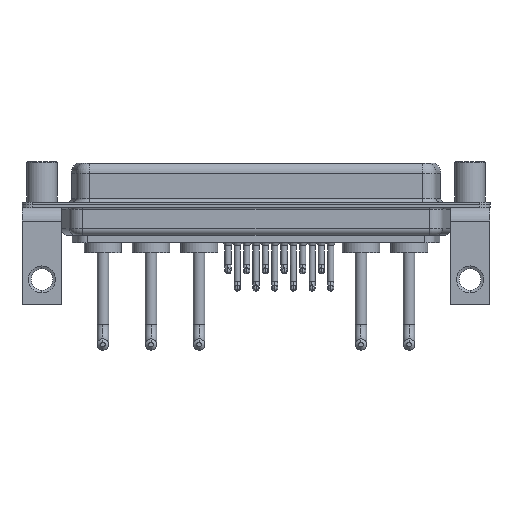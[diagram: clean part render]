
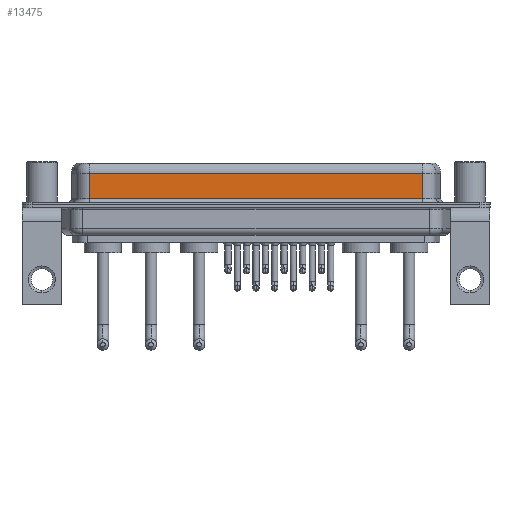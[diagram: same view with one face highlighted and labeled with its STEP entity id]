
A CAD part, front view. The second image highlights one B-rep face of the part: STEP entity #13475.
In plain terms, the highlighted planar face has unit normal (0, -1, 0).
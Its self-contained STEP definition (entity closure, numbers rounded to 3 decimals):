
#339 = VERTEX_POINT ( 'NONE', #3118 ) ;
#616 = DIRECTION ( 'NONE',  ( -1., 0., 0. ) ) ;
#667 = ORIENTED_EDGE ( 'NONE', *, *, #9464, .T. ) ;
#1464 = VECTOR ( 'NONE', #3838, 1000. ) ;
#2189 = LINE ( 'NONE', #9022, #3500 ) ;
#2222 = EDGE_CURVE ( 'NONE', #6596, #19165, #9717, .T. ) ;
#2508 = AXIS2_PLACEMENT_3D ( 'NONE', #5162, #19135, #3437 ) ;
#3118 = CARTESIAN_POINT ( 'NONE',  ( 7.038, -3.95, 4.65 ) ) ;
#3431 = EDGE_CURVE ( 'NONE', #14844, #19165, #19658, .T. ) ;
#3437 = DIRECTION ( 'NONE',  ( 0., 0., 1. ) ) ;
#3500 = VECTOR ( 'NONE', #616, 1000. ) ;
#3838 = DIRECTION ( 'NONE',  ( 1., 0., 0. ) ) ;
#5162 = CARTESIAN_POINT ( 'NONE',  ( 56.462, -3.95, 6.4 ) ) ;
#6596 = VERTEX_POINT ( 'NONE', #10594 ) ;
#6898 = CARTESIAN_POINT ( 'NONE',  ( 7.038, -3.95, 0.9 ) ) ;
#7156 = EDGE_LOOP ( 'NONE', ( #17201, #18753, #667, #19845 ) ) ;
#8074 = EDGE_CURVE ( 'NONE', #6596, #339, #2189, .T. ) ;
#9022 = CARTESIAN_POINT ( 'NONE',  ( 56.462, -3.95, 4.65 ) ) ;
#9261 = LINE ( 'NONE', #10861, #20850 ) ;
#9464 = EDGE_CURVE ( 'NONE', #339, #14844, #9261, .T. ) ;
#9717 = LINE ( 'NONE', #16739, #19604 ) ;
#10594 = CARTESIAN_POINT ( 'NONE',  ( 56.462, -3.95, 4.65 ) ) ;
#10861 = CARTESIAN_POINT ( 'NONE',  ( 7.038, -3.95, 6.4 ) ) ;
#12096 = PLANE ( 'NONE',  #2508 ) ;
#12380 = CARTESIAN_POINT ( 'NONE',  ( 56.462, -3.95, 0.9 ) ) ;
#13072 = DIRECTION ( 'NONE',  ( 0., 0., -1. ) ) ;
#13475 = ADVANCED_FACE ( 'NONE', ( #21288 ), #12096, .F. ) ;
#14844 = VERTEX_POINT ( 'NONE', #6898 ) ;
#16739 = CARTESIAN_POINT ( 'NONE',  ( 56.462, -3.95, 6.4 ) ) ;
#17201 = ORIENTED_EDGE ( 'NONE', *, *, #2222, .F. ) ;
#17904 = DIRECTION ( 'NONE',  ( 0., 0., -1. ) ) ;
#18682 = CARTESIAN_POINT ( 'NONE',  ( 56.462, -3.95, 0.9 ) ) ;
#18753 = ORIENTED_EDGE ( 'NONE', *, *, #8074, .T. ) ;
#19135 = DIRECTION ( 'NONE',  ( 0., 1., 0. ) ) ;
#19165 = VERTEX_POINT ( 'NONE', #18682 ) ;
#19604 = VECTOR ( 'NONE', #13072, 1000. ) ;
#19658 = LINE ( 'NONE', #12380, #1464 ) ;
#19845 = ORIENTED_EDGE ( 'NONE', *, *, #3431, .T. ) ;
#20850 = VECTOR ( 'NONE', #17904, 1000. ) ;
#21288 = FACE_OUTER_BOUND ( 'NONE', #7156, .T. ) ;
